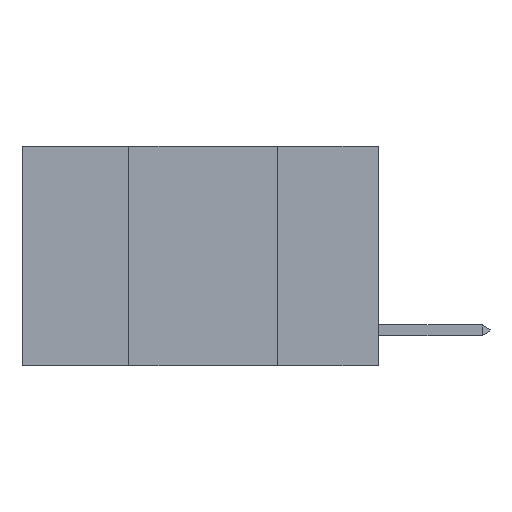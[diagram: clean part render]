
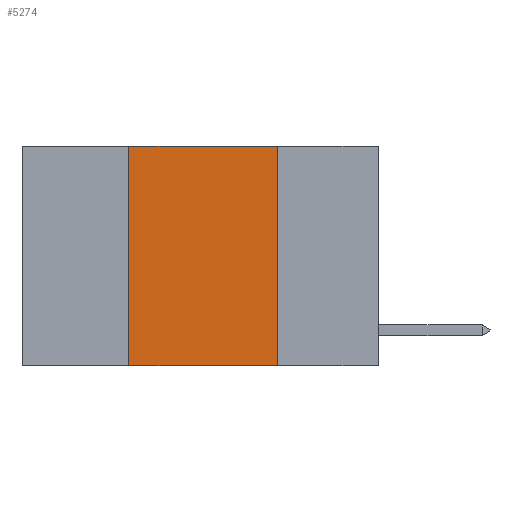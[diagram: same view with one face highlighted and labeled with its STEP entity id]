
A CAD part, left-side view. The second image highlights one B-rep face of the part: STEP entity #5274.
In plain terms, the highlighted planar face has unit normal (-1, 0, 0).
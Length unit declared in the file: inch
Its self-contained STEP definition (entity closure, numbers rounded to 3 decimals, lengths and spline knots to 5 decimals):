
#1529 = CARTESIAN_POINT ( 'NONE',  ( 0., 0.6, -0.37 ) ) ;
#1733 = EDGE_CURVE ( 'NONE', #9776, #5595, #9247, .T. ) ;
#1958 = EDGE_CURVE ( 'NONE', #5927, #9776, #7764, .T. ) ;
#2179 = VERTEX_POINT ( 'NONE', #4847 ) ;
#2271 = DIRECTION ( 'NONE',  ( 0., 0., -1. ) ) ;
#2735 = ORIENTED_EDGE ( 'NONE', *, *, #1958, .F. ) ;
#3050 = AXIS2_PLACEMENT_3D ( 'NONE', #11680, #3175, #2271 ) ;
#3175 = DIRECTION ( 'NONE',  ( 1., 0., 0. ) ) ;
#3345 = EDGE_CURVE ( 'NONE', #5595, #2179, #10968, .T. ) ;
#3688 = CARTESIAN_POINT ( 'NONE',  ( 0., 0.42, -0.37 ) ) ;
#3765 = VECTOR ( 'NONE', #7699, 39.37008 ) ;
#4381 = EDGE_LOOP ( 'NONE', ( #8250, #12007, #2735, #11419 ) ) ;
#4847 = CARTESIAN_POINT ( 'NONE',  ( 0., 0.17, -0.37 ) ) ;
#5274 = ADVANCED_FACE ( 'NONE', ( #11061 ), #6921, .F. ) ;
#5595 = VERTEX_POINT ( 'NONE', #11378 ) ;
#5927 = VERTEX_POINT ( 'NONE', #3688 ) ;
#5966 = VECTOR ( 'NONE', #7377, 39.37008 ) ;
#6547 = EDGE_CURVE ( 'NONE', #5927, #2179, #8416, .T. ) ;
#6749 = DIRECTION ( 'NONE',  ( 0., 0., -1. ) ) ;
#6921 = PLANE ( 'NONE',  #3050 ) ;
#7268 = CARTESIAN_POINT ( 'NONE',  ( 0., 0.42, 0. ) ) ;
#7377 = DIRECTION ( 'NONE',  ( 0., -1., 0. ) ) ;
#7415 = CARTESIAN_POINT ( 'NONE',  ( 0., 0.6, 0. ) ) ;
#7699 = DIRECTION ( 'NONE',  ( 0., 0., 1. ) ) ;
#7764 = LINE ( 'NONE', #7852, #3765 ) ;
#7852 = CARTESIAN_POINT ( 'NONE',  ( 0., 0.42, 0. ) ) ;
#8250 = ORIENTED_EDGE ( 'NONE', *, *, #3345, .F. ) ;
#8416 = LINE ( 'NONE', #1529, #9738 ) ;
#9042 = DIRECTION ( 'NONE',  ( 0., -1., 0. ) ) ;
#9247 = LINE ( 'NONE', #7415, #5966 ) ;
#9249 = CARTESIAN_POINT ( 'NONE',  ( 0., 0.17, 0. ) ) ;
#9527 = VECTOR ( 'NONE', #6749, 39.37008 ) ;
#9738 = VECTOR ( 'NONE', #9042, 39.37008 ) ;
#9776 = VERTEX_POINT ( 'NONE', #7268 ) ;
#10968 = LINE ( 'NONE', #9249, #9527 ) ;
#11061 = FACE_OUTER_BOUND ( 'NONE', #4381, .T. ) ;
#11378 = CARTESIAN_POINT ( 'NONE',  ( 0., 0.17, 0. ) ) ;
#11419 = ORIENTED_EDGE ( 'NONE', *, *, #6547, .T. ) ;
#11680 = CARTESIAN_POINT ( 'NONE',  ( 0., 0.6, 0. ) ) ;
#12007 = ORIENTED_EDGE ( 'NONE', *, *, #1733, .F. ) ;
